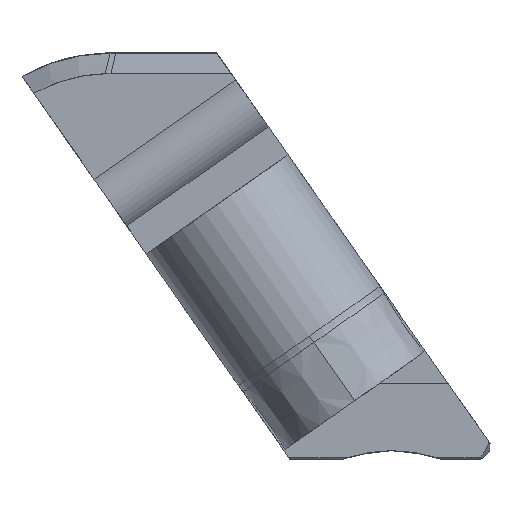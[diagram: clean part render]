
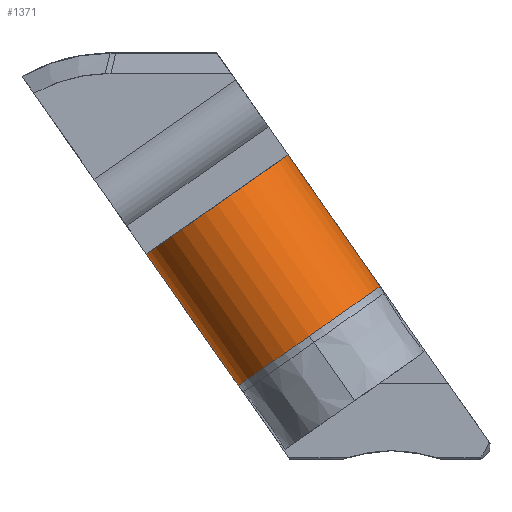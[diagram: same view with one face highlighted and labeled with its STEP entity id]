
A CAD part, left-side view. The second image highlights one B-rep face of the part: STEP entity #1371.
In plain terms, the highlighted cylindrical face has radius 2.14 mm (diameter 4.28 mm), a partial arc.
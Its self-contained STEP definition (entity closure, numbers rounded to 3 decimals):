
#38 = CARTESIAN_POINT ( 'NONE',  ( -25.864, -1.351, 10.864 ) ) ;
#87 = AXIS2_PLACEMENT_3D ( 'NONE', #970, #1412, #2344 ) ;
#98 = VECTOR ( 'NONE', #1655, 1000. ) ;
#101 = DIRECTION ( 'NONE',  ( 0., 0.574, 0.819 ) ) ;
#179 = FACE_OUTER_BOUND ( 'NONE', #813, .T. ) ;
#218 = VERTEX_POINT ( 'NONE', #2039 ) ;
#330 = CARTESIAN_POINT ( 'NONE',  ( -28.003, -1.877, 6.381 ) ) ;
#381 = DIRECTION ( 'NONE',  ( 0., -0.574, -0.819 ) ) ;
#486 = ORIENTED_EDGE ( 'NONE', *, *, #2540, .F. ) ;
#518 = CARTESIAN_POINT ( 'NONE',  ( -25.864, -1.351, 10.864 ) ) ;
#737 = LINE ( 'NONE', #1881, #98 ) ;
#763 = AXIS2_PLACEMENT_3D ( 'NONE', #1747, #381, #1981 ) ;
#770 = CARTESIAN_POINT ( 'NONE',  ( -25.864, 2.155, 8.409 ) ) ;
#793 = CIRCLE ( 'NONE', #1024, 2.14 ) ;
#813 = EDGE_LOOP ( 'NONE', ( #486, #2215, #2957, #1349, #2671 ) ) ;
#970 = CARTESIAN_POINT ( 'NONE',  ( -25.864, 0.402, 9.636 ) ) ;
#1024 = AXIS2_PLACEMENT_3D ( 'NONE', #2567, #1202, #2799 ) ;
#1159 = CIRCLE ( 'NONE', #763, 2.14 ) ;
#1202 = DIRECTION ( 'NONE',  ( 0., -0.574, -0.819 ) ) ;
#1289 = VECTOR ( 'NONE', #2362, 1000. ) ;
#1349 = ORIENTED_EDGE ( 'NONE', *, *, #2254, .F. ) ;
#1371 = ADVANCED_FACE ( 'NONE', ( #179 ), #1946, .T. ) ;
#1399 = EDGE_CURVE ( 'NONE', #1518, #218, #737, .T. ) ;
#1412 = DIRECTION ( 'NONE',  ( 0., -0.574, -0.819 ) ) ;
#1413 = VERTEX_POINT ( 'NONE', #38 ) ;
#1492 = CARTESIAN_POINT ( 'NONE',  ( -25.864, 0.402, 9.636 ) ) ;
#1518 = VERTEX_POINT ( 'NONE', #770 ) ;
#1544 = VERTEX_POINT ( 'NONE', #330 ) ;
#1655 = DIRECTION ( 'NONE',  ( 0., -0.574, -0.819 ) ) ;
#1716 = CIRCLE ( 'NONE', #2665, 2.14 ) ;
#1720 = DIRECTION ( 'NONE',  ( 0., 0.819, -0.574 ) ) ;
#1747 = CARTESIAN_POINT ( 'NONE',  ( -25.864, -1.877, 6.381 ) ) ;
#1855 = EDGE_CURVE ( 'NONE', #1518, #1413, #1716, .T. ) ;
#1866 = CARTESIAN_POINT ( 'NONE',  ( -25.864, -3.63, 7.608 ) ) ;
#1881 = CARTESIAN_POINT ( 'NONE',  ( -25.864, 2.155, 8.409 ) ) ;
#1946 = CYLINDRICAL_SURFACE ( 'NONE', #87, 2.14 ) ;
#1981 = DIRECTION ( 'NONE',  ( 0., 0.819, -0.574 ) ) ;
#2039 = CARTESIAN_POINT ( 'NONE',  ( -25.864, -0.124, 5.153 ) ) ;
#2074 = EDGE_CURVE ( 'NONE', #2253, #1544, #1159, .T. ) ;
#2215 = ORIENTED_EDGE ( 'NONE', *, *, #1855, .F. ) ;
#2253 = VERTEX_POINT ( 'NONE', #1866 ) ;
#2254 = EDGE_CURVE ( 'NONE', #1544, #218, #793, .T. ) ;
#2344 = DIRECTION ( 'NONE',  ( 0., 0.819, -0.574 ) ) ;
#2362 = DIRECTION ( 'NONE',  ( 0., -0.574, -0.819 ) ) ;
#2511 = LINE ( 'NONE', #518, #1289 ) ;
#2540 = EDGE_CURVE ( 'NONE', #1413, #2253, #2511, .T. ) ;
#2567 = CARTESIAN_POINT ( 'NONE',  ( -25.864, -1.877, 6.381 ) ) ;
#2665 = AXIS2_PLACEMENT_3D ( 'NONE', #1492, #101, #1720 ) ;
#2671 = ORIENTED_EDGE ( 'NONE', *, *, #2074, .F. ) ;
#2799 = DIRECTION ( 'NONE',  ( 0., 0.819, -0.574 ) ) ;
#2957 = ORIENTED_EDGE ( 'NONE', *, *, #1399, .T. ) ;
